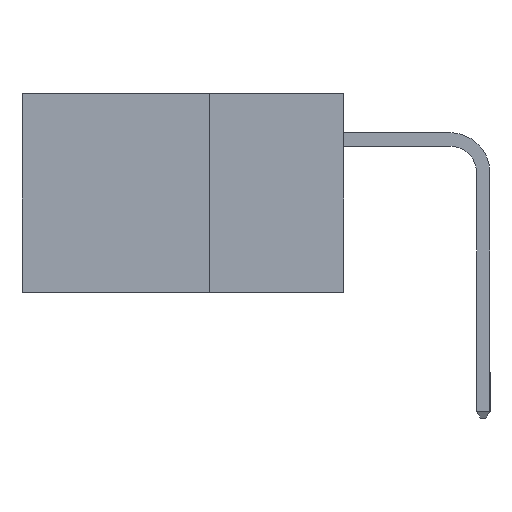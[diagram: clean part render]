
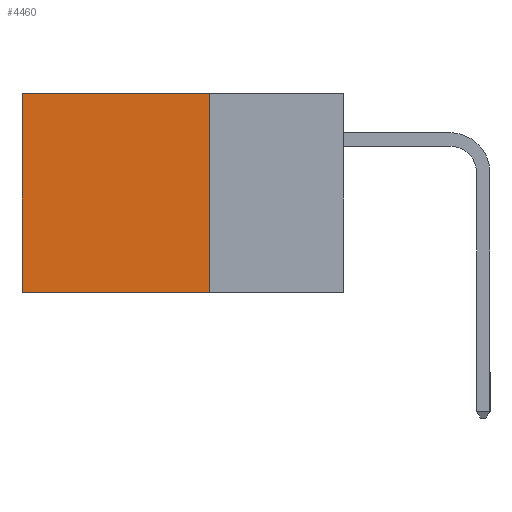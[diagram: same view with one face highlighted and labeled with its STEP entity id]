
A CAD part, left-side view. The second image highlights one B-rep face of the part: STEP entity #4460.
In plain terms, the highlighted planar face has unit normal (-1, 0, 0).
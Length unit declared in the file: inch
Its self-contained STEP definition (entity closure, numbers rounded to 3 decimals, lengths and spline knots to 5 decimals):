
#537 = VERTEX_POINT ( 'NONE', #6754 ) ;
#674 = FACE_OUTER_BOUND ( 'NONE', #21765, .T. ) ;
#3211 = ORIENTED_EDGE ( 'NONE', *, *, #8294, .T. ) ;
#4038 = VERTEX_POINT ( 'NONE', #8217 ) ;
#4460 = ADVANCED_FACE ( 'NONE', ( #674 ), #5333, .F. ) ;
#5333 = PLANE ( 'NONE',  #24184 ) ;
#6160 = ORIENTED_EDGE ( 'NONE', *, *, #14416, .T. ) ;
#6272 = CARTESIAN_POINT ( 'NONE',  ( 0.298, 0.25, 0. ) ) ;
#6754 = CARTESIAN_POINT ( 'NONE',  ( 0.298, 0.6, 0. ) ) ;
#7346 = CARTESIAN_POINT ( 'NONE',  ( 0.298, 0.25, 0. ) ) ;
#8217 = CARTESIAN_POINT ( 'NONE',  ( 0.298, 0.6, -0.37 ) ) ;
#8294 = EDGE_CURVE ( 'NONE', #13662, #537, #25540, .T. ) ;
#8489 = EDGE_CURVE ( 'NONE', #10969, #4038, #20058, .T. ) ;
#9001 = EDGE_CURVE ( 'NONE', #13662, #10969, #20361, .T. ) ;
#9170 = VECTOR ( 'NONE', #20663, 39.37008 ) ;
#10290 = DIRECTION ( 'NONE',  ( 0., 0., -1. ) ) ;
#10969 = VERTEX_POINT ( 'NONE', #13250 ) ;
#11483 = CARTESIAN_POINT ( 'NONE',  ( 0.298, 0.6, 0. ) ) ;
#13250 = CARTESIAN_POINT ( 'NONE',  ( 0.298, 0.25, -0.37 ) ) ;
#13662 = VERTEX_POINT ( 'NONE', #25773 ) ;
#14231 = CARTESIAN_POINT ( 'NONE',  ( 0.298, 0.25, 0. ) ) ;
#14416 = EDGE_CURVE ( 'NONE', #537, #4038, #17937, .T. ) ;
#14611 = DIRECTION ( 'NONE',  ( 1., 0., 0. ) ) ;
#17489 = ORIENTED_EDGE ( 'NONE', *, *, #9001, .F. ) ;
#17937 = LINE ( 'NONE', #11483, #20989 ) ;
#20058 = LINE ( 'NONE', #24940, #9170 ) ;
#20361 = LINE ( 'NONE', #6272, #26816 ) ;
#20468 = DIRECTION ( 'NONE',  ( 0., 1., 0. ) ) ;
#20663 = DIRECTION ( 'NONE',  ( 0., 1., 0. ) ) ;
#20989 = VECTOR ( 'NONE', #24577, 39.37008 ) ;
#21197 = DIRECTION ( 'NONE',  ( 0., 0., -1. ) ) ;
#21765 = EDGE_LOOP ( 'NONE', ( #6160, #27287, #17489, #3211 ) ) ;
#22119 = VECTOR ( 'NONE', #20468, 39.37008 ) ;
#24184 = AXIS2_PLACEMENT_3D ( 'NONE', #14231, #14611, #10290 ) ;
#24577 = DIRECTION ( 'NONE',  ( 0., 0., -1. ) ) ;
#24940 = CARTESIAN_POINT ( 'NONE',  ( 0.298, 0.25, -0.37 ) ) ;
#25540 = LINE ( 'NONE', #7346, #22119 ) ;
#25773 = CARTESIAN_POINT ( 'NONE',  ( 0.298, 0.25, 0. ) ) ;
#26816 = VECTOR ( 'NONE', #21197, 39.37008 ) ;
#27287 = ORIENTED_EDGE ( 'NONE', *, *, #8489, .F. ) ;
